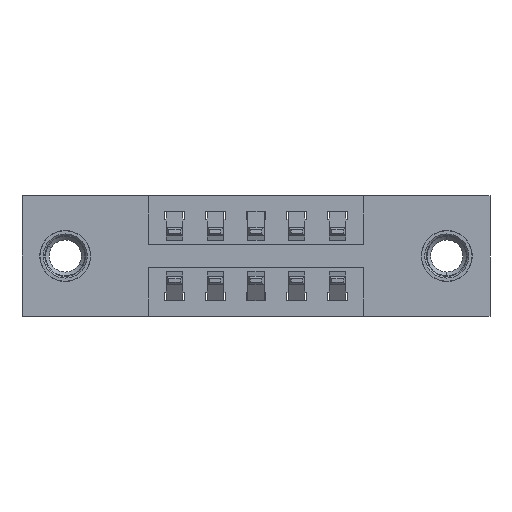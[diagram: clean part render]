
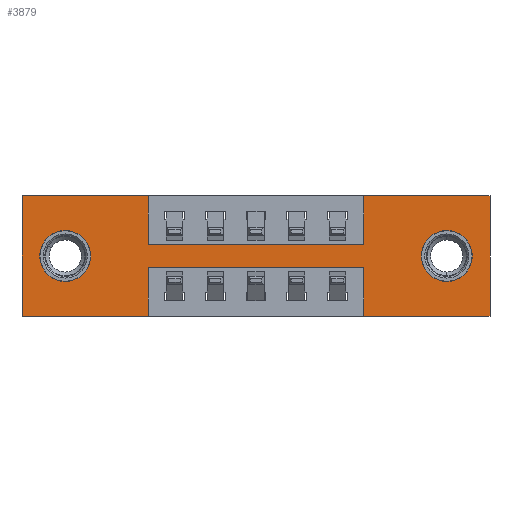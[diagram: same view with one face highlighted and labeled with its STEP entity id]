
A CAD part, front view. The second image highlights one B-rep face of the part: STEP entity #3879.
In plain terms, the highlighted planar face has unit normal (0, -1, 0).
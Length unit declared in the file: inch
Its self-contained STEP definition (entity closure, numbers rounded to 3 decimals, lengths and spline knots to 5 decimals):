
#41 = LINE ( 'NONE', #9531, #8062 ) ;
#63 = DIRECTION ( 'NONE',  ( 0., 0., -1. ) ) ;
#160 = EDGE_CURVE ( 'NONE', #2250, #684, #5955, .T. ) ;
#188 = VECTOR ( 'NONE', #9089, 39.37008 ) ;
#210 = CARTESIAN_POINT ( 'NONE',  ( 0., 0., -0.37 ) ) ;
#342 = VECTOR ( 'NONE', #8175, 39.37008 ) ;
#410 = LINE ( 'NONE', #8308, #342 ) ;
#607 = EDGE_CURVE ( 'NONE', #684, #2250, #7348, .T. ) ;
#684 = VERTEX_POINT ( 'NONE', #6139 ) ;
#754 = AXIS2_PLACEMENT_3D ( 'NONE', #8995, #8799, #8913 ) ;
#948 = VERTEX_POINT ( 'NONE', #1197 ) ;
#974 = DIRECTION ( 'NONE',  ( -1., 0., 0. ) ) ;
#1197 = CARTESIAN_POINT ( 'NONE',  ( 1.435, 0., 0. ) ) ;
#1358 = EDGE_CURVE ( 'NONE', #1401, #8832, #6666, .T. ) ;
#1401 = VERTEX_POINT ( 'NONE', #6238 ) ;
#1439 = ORIENTED_EDGE ( 'NONE', *, *, #4406, .T. ) ;
#1507 = ORIENTED_EDGE ( 'NONE', *, *, #2764, .F. ) ;
#1956 = VERTEX_POINT ( 'NONE', #4077 ) ;
#2005 = ORIENTED_EDGE ( 'NONE', *, *, #607, .T. ) ;
#2023 = LINE ( 'NONE', #6319, #9467 ) ;
#2250 = VERTEX_POINT ( 'NONE', #5266 ) ;
#2260 = ORIENTED_EDGE ( 'NONE', *, *, #8593, .F. ) ;
#2313 = EDGE_CURVE ( 'NONE', #5902, #3262, #410, .T. ) ;
#2538 = LINE ( 'NONE', #6561, #5914 ) ;
#2677 = CARTESIAN_POINT ( 'NONE',  ( 0., 0., -0.37 ) ) ;
#2702 = CARTESIAN_POINT ( 'NONE',  ( 0., 0., 0. ) ) ;
#2764 = EDGE_CURVE ( 'NONE', #948, #6086, #2538, .T. ) ;
#2875 = VECTOR ( 'NONE', #9538, 39.37008 ) ;
#3008 = EDGE_CURVE ( 'NONE', #4313, #1956, #9249, .T. ) ;
#3131 = VECTOR ( 'NONE', #3531, 39.37008 ) ;
#3262 = VERTEX_POINT ( 'NONE', #8515 ) ;
#3361 = CARTESIAN_POINT ( 'NONE',  ( 1.0475, 0., 0. ) ) ;
#3492 = EDGE_LOOP ( 'NONE', ( #9062, #2005 ) ) ;
#3531 = DIRECTION ( 'NONE',  ( -1., 0., 0. ) ) ;
#3561 = ORIENTED_EDGE ( 'NONE', *, *, #2313, .F. ) ;
#3613 = EDGE_CURVE ( 'NONE', #8832, #6003, #7451, .T. ) ;
#3615 = CARTESIAN_POINT ( 'NONE',  ( 1.3025, 0., -0.263 ) ) ;
#3659 = ORIENTED_EDGE ( 'NONE', *, *, #4325, .F. ) ;
#3879 = ADVANCED_FACE ( 'NONE', ( #5786, #9160, #4072 ), #7641, .T. ) ;
#3961 = VECTOR ( 'NONE', #9489, 39.37008 ) ;
#4072 = FACE_OUTER_BOUND ( 'NONE', #4702, .T. ) ;
#4077 = CARTESIAN_POINT ( 'NONE',  ( 0.3875, 0., 0. ) ) ;
#4173 = LINE ( 'NONE', #7635, #7629 ) ;
#4175 = ORIENTED_EDGE ( 'NONE', *, *, #8622, .F. ) ;
#4313 = VERTEX_POINT ( 'NONE', #2702 ) ;
#4325 = EDGE_CURVE ( 'NONE', #3262, #4601, #8701, .T. ) ;
#4353 = VERTEX_POINT ( 'NONE', #3615 ) ;
#4406 = EDGE_CURVE ( 'NONE', #4451, #4353, #5457, .T. ) ;
#4437 = AXIS2_PLACEMENT_3D ( 'NONE', #5382, #5059, #5485 ) ;
#4451 = VERTEX_POINT ( 'NONE', #4769 ) ;
#4496 = CIRCLE ( 'NONE', #7651, 0.078 ) ;
#4572 = ORIENTED_EDGE ( 'NONE', *, *, #7849, .F. ) ;
#4601 = VERTEX_POINT ( 'NONE', #7012 ) ;
#4702 = EDGE_LOOP ( 'NONE', ( #8591, #3659, #3561, #2260, #1507, #4175, #7491, #7266, #4572, #6210, #6270, #6429 ) ) ;
#4769 = CARTESIAN_POINT ( 'NONE',  ( 1.3025, 0., -0.107 ) ) ;
#4878 = EDGE_CURVE ( 'NONE', #6346, #4313, #41, .T. ) ;
#4947 = LINE ( 'NONE', #5094, #2875 ) ;
#4991 = EDGE_CURVE ( 'NONE', #5721, #6346, #4173, .T. ) ;
#5059 = DIRECTION ( 'NONE',  ( 0., 1., 0. ) ) ;
#5094 = CARTESIAN_POINT ( 'NONE',  ( 0., 0., 0. ) ) ;
#5175 = DIRECTION ( 'NONE',  ( 0., 1., 0. ) ) ;
#5266 = CARTESIAN_POINT ( 'NONE',  ( 0.1325, 0., -0.107 ) ) ;
#5285 = CARTESIAN_POINT ( 'NONE',  ( 0., 0., 0. ) ) ;
#5317 = CARTESIAN_POINT ( 'NONE',  ( 1.435, 0., -0.37 ) ) ;
#5324 = AXIS2_PLACEMENT_3D ( 'NONE', #7516, #7503, #7495 ) ;
#5382 = CARTESIAN_POINT ( 'NONE',  ( 1.3025, 0., -0.185 ) ) ;
#5457 = CIRCLE ( 'NONE', #4437, 0.078 ) ;
#5485 = DIRECTION ( 'NONE',  ( 0., 0., -1. ) ) ;
#5721 = VERTEX_POINT ( 'NONE', #6087 ) ;
#5786 = FACE_BOUND ( 'NONE', #9497, .T. ) ;
#5851 = EDGE_CURVE ( 'NONE', #4601, #5721, #8146, .T. ) ;
#5902 = VERTEX_POINT ( 'NONE', #8133 ) ;
#5914 = VECTOR ( 'NONE', #9304, 39.37008 ) ;
#5955 = CIRCLE ( 'NONE', #754, 0.078 ) ;
#6003 = VERTEX_POINT ( 'NONE', #6603 ) ;
#6086 = VERTEX_POINT ( 'NONE', #5317 ) ;
#6087 = CARTESIAN_POINT ( 'NONE',  ( 0.3875, 0., -0.37 ) ) ;
#6139 = CARTESIAN_POINT ( 'NONE',  ( 0.1325, 0., -0.263 ) ) ;
#6210 = ORIENTED_EDGE ( 'NONE', *, *, #3008, .F. ) ;
#6238 = CARTESIAN_POINT ( 'NONE',  ( 0.3875, 0., -0.15 ) ) ;
#6270 = ORIENTED_EDGE ( 'NONE', *, *, #4878, .F. ) ;
#6319 = CARTESIAN_POINT ( 'NONE',  ( 0.3875, 0., 0. ) ) ;
#6346 = VERTEX_POINT ( 'NONE', #210 ) ;
#6374 = DIRECTION ( 'NONE',  ( 0., 0., 1. ) ) ;
#6429 = ORIENTED_EDGE ( 'NONE', *, *, #4991, .F. ) ;
#6561 = CARTESIAN_POINT ( 'NONE',  ( 1.435, 0., 0. ) ) ;
#6603 = CARTESIAN_POINT ( 'NONE',  ( 1.0475, 0., 0. ) ) ;
#6666 = LINE ( 'NONE', #7722, #7610 ) ;
#6737 = ORIENTED_EDGE ( 'NONE', *, *, #9417, .T. ) ;
#6909 = AXIS2_PLACEMENT_3D ( 'NONE', #7693, #7126, #7122 ) ;
#6914 = CARTESIAN_POINT ( 'NONE',  ( 0.3875, 0., -0.22 ) ) ;
#7012 = CARTESIAN_POINT ( 'NONE',  ( 0.3875, 0., -0.22 ) ) ;
#7020 = VECTOR ( 'NONE', #974, 39.37008 ) ;
#7122 = DIRECTION ( 'NONE',  ( 0., 0., -1. ) ) ;
#7126 = DIRECTION ( 'NONE',  ( 0., -1., 0. ) ) ;
#7266 = ORIENTED_EDGE ( 'NONE', *, *, #1358, .F. ) ;
#7303 = CARTESIAN_POINT ( 'NONE',  ( 1.0475, 0., -0.15 ) ) ;
#7348 = CIRCLE ( 'NONE', #5324, 0.078 ) ;
#7451 = LINE ( 'NONE', #3361, #8898 ) ;
#7491 = ORIENTED_EDGE ( 'NONE', *, *, #3613, .F. ) ;
#7495 = DIRECTION ( 'NONE',  ( 0., 0., 1. ) ) ;
#7503 = DIRECTION ( 'NONE',  ( 0., 1., 0. ) ) ;
#7516 = CARTESIAN_POINT ( 'NONE',  ( 0.1325, 0., -0.185 ) ) ;
#7525 = DIRECTION ( 'NONE',  ( 1., 0., 0. ) ) ;
#7610 = VECTOR ( 'NONE', #7525, 39.37008 ) ;
#7629 = VECTOR ( 'NONE', #7895, 39.37008 ) ;
#7635 = CARTESIAN_POINT ( 'NONE',  ( 0., 0., -0.37 ) ) ;
#7641 = PLANE ( 'NONE',  #6909 ) ;
#7651 = AXIS2_PLACEMENT_3D ( 'NONE', #9047, #5175, #63 ) ;
#7693 = CARTESIAN_POINT ( 'NONE',  ( 0., 0., -0.37 ) ) ;
#7722 = CARTESIAN_POINT ( 'NONE',  ( 0.3875, 0., -0.15 ) ) ;
#7849 = EDGE_CURVE ( 'NONE', #1956, #1401, #2023, .T. ) ;
#7895 = DIRECTION ( 'NONE',  ( -1., 0., 0. ) ) ;
#8062 = VECTOR ( 'NONE', #9345, 39.37008 ) ;
#8133 = CARTESIAN_POINT ( 'NONE',  ( 1.0475, 0., -0.37 ) ) ;
#8146 = LINE ( 'NONE', #9100, #188 ) ;
#8175 = DIRECTION ( 'NONE',  ( 0., 0., 1. ) ) ;
#8308 = CARTESIAN_POINT ( 'NONE',  ( 1.0475, 0., -0.37 ) ) ;
#8515 = CARTESIAN_POINT ( 'NONE',  ( 1.0475, 0., -0.22 ) ) ;
#8591 = ORIENTED_EDGE ( 'NONE', *, *, #5851, .F. ) ;
#8593 = EDGE_CURVE ( 'NONE', #6086, #5902, #8847, .T. ) ;
#8622 = EDGE_CURVE ( 'NONE', #6003, #948, #4947, .T. ) ;
#8701 = LINE ( 'NONE', #6914, #7020 ) ;
#8799 = DIRECTION ( 'NONE',  ( 0., 1., 0. ) ) ;
#8832 = VERTEX_POINT ( 'NONE', #7303 ) ;
#8847 = LINE ( 'NONE', #2677, #3131 ) ;
#8898 = VECTOR ( 'NONE', #6374, 39.37008 ) ;
#8913 = DIRECTION ( 'NONE',  ( 0., 0., 1. ) ) ;
#8995 = CARTESIAN_POINT ( 'NONE',  ( 0.1325, 0., -0.185 ) ) ;
#9047 = CARTESIAN_POINT ( 'NONE',  ( 1.3025, 0., -0.185 ) ) ;
#9062 = ORIENTED_EDGE ( 'NONE', *, *, #160, .T. ) ;
#9089 = DIRECTION ( 'NONE',  ( 0., 0., -1. ) ) ;
#9100 = CARTESIAN_POINT ( 'NONE',  ( 0.3875, 0., -0.37 ) ) ;
#9160 = FACE_BOUND ( 'NONE', #3492, .T. ) ;
#9249 = LINE ( 'NONE', #5285, #3961 ) ;
#9304 = DIRECTION ( 'NONE',  ( 0., 0., -1. ) ) ;
#9345 = DIRECTION ( 'NONE',  ( 0., 0., 1. ) ) ;
#9417 = EDGE_CURVE ( 'NONE', #4353, #4451, #4496, .T. ) ;
#9445 = DIRECTION ( 'NONE',  ( 0., 0., -1. ) ) ;
#9467 = VECTOR ( 'NONE', #9445, 39.37008 ) ;
#9489 = DIRECTION ( 'NONE',  ( 1., 0., 0. ) ) ;
#9497 = EDGE_LOOP ( 'NONE', ( #1439, #6737 ) ) ;
#9531 = CARTESIAN_POINT ( 'NONE',  ( 0., 0., 0. ) ) ;
#9538 = DIRECTION ( 'NONE',  ( 1., 0., 0. ) ) ;
